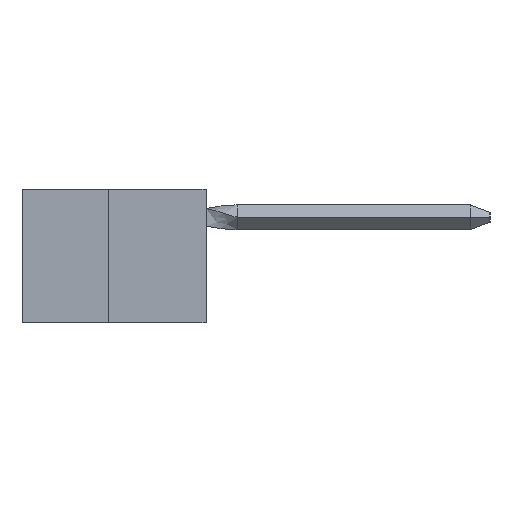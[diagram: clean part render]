
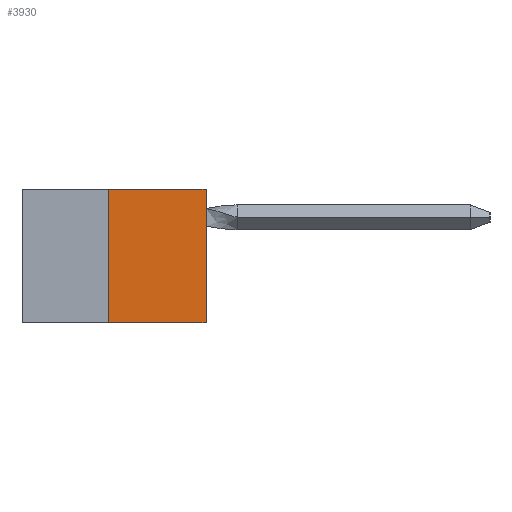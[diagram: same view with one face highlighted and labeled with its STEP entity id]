
A CAD part, left-side view. The second image highlights one B-rep face of the part: STEP entity #3930.
In plain terms, the highlighted planar face has unit normal (-1, 0, 0).
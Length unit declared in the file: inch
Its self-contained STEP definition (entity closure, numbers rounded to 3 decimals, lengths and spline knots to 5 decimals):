
#217 = PLANE ( 'NONE',  #3294 ) ;
#584 = VECTOR ( 'NONE', #3370, 39.37008 ) ;
#768 = CARTESIAN_POINT ( 'NONE',  ( 0., 0.473, -0.343 ) ) ;
#1749 = LINE ( 'NONE', #768, #3375 ) ;
#3141 = CARTESIAN_POINT ( 'NONE',  ( 0., 0.25, 0. ) ) ;
#3294 = AXIS2_PLACEMENT_3D ( 'NONE', #15973, #21239, #10775 ) ;
#3370 = DIRECTION ( 'NONE',  ( 0., 0., 1. ) ) ;
#3375 = VECTOR ( 'NONE', #21808, 39.37008 ) ;
#3505 = ORIENTED_EDGE ( 'NONE', *, *, #8114, .F. ) ;
#3748 = DIRECTION ( 'NONE',  ( 0., 0., 1. ) ) ;
#3921 = EDGE_CURVE ( 'NONE', #8019, #22308, #10177, .T. ) ;
#3930 = ADVANCED_FACE ( 'NONE', ( #8537 ), #217, .F. ) ;
#4022 = ORIENTED_EDGE ( 'NONE', *, *, #3921, .T. ) ;
#4429 = VECTOR ( 'NONE', #3748, 39.37008 ) ;
#5158 = CARTESIAN_POINT ( 'NONE',  ( 0., 0., -0.343 ) ) ;
#5564 = CARTESIAN_POINT ( 'NONE',  ( 0., 0., 0. ) ) ;
#6681 = EDGE_CURVE ( 'NONE', #21767, #8019, #1749, .T. ) ;
#6831 = LINE ( 'NONE', #17158, #584 ) ;
#8019 = VERTEX_POINT ( 'NONE', #5158 ) ;
#8114 = EDGE_CURVE ( 'NONE', #21767, #9805, #6831, .T. ) ;
#8537 = FACE_OUTER_BOUND ( 'NONE', #11643, .T. ) ;
#8938 = CARTESIAN_POINT ( 'NONE',  ( 0., 0.473, 0. ) ) ;
#9464 = CARTESIAN_POINT ( 'NONE',  ( 0., 0., 0. ) ) ;
#9489 = CARTESIAN_POINT ( 'NONE',  ( 0., 0.25, -0.343 ) ) ;
#9805 = VERTEX_POINT ( 'NONE', #3141 ) ;
#10177 = LINE ( 'NONE', #5564, #4429 ) ;
#10353 = LINE ( 'NONE', #8938, #19093 ) ;
#10423 = ORIENTED_EDGE ( 'NONE', *, *, #16320, .F. ) ;
#10775 = DIRECTION ( 'NONE',  ( 0., 0., -1. ) ) ;
#11643 = EDGE_LOOP ( 'NONE', ( #10423, #3505, #16311, #4022 ) ) ;
#12377 = DIRECTION ( 'NONE',  ( 0., -1., 0. ) ) ;
#15973 = CARTESIAN_POINT ( 'NONE',  ( 0., 0.473, 0. ) ) ;
#16311 = ORIENTED_EDGE ( 'NONE', *, *, #6681, .T. ) ;
#16320 = EDGE_CURVE ( 'NONE', #9805, #22308, #10353, .T. ) ;
#17158 = CARTESIAN_POINT ( 'NONE',  ( 0., 0.25, 0. ) ) ;
#19093 = VECTOR ( 'NONE', #12377, 39.37008 ) ;
#21239 = DIRECTION ( 'NONE',  ( 1., 0., 0. ) ) ;
#21767 = VERTEX_POINT ( 'NONE', #9489 ) ;
#21808 = DIRECTION ( 'NONE',  ( 0., -1., 0. ) ) ;
#22308 = VERTEX_POINT ( 'NONE', #9464 ) ;
